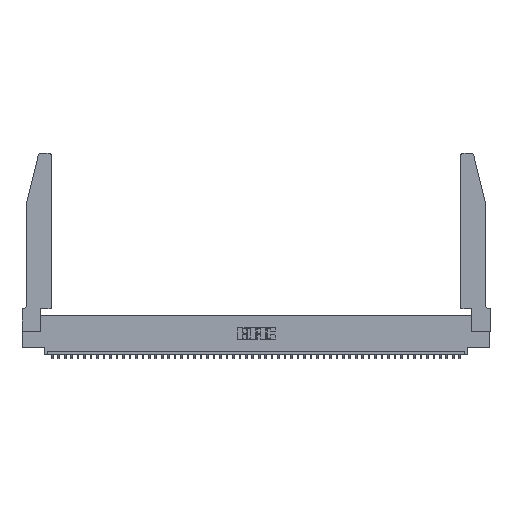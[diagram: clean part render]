
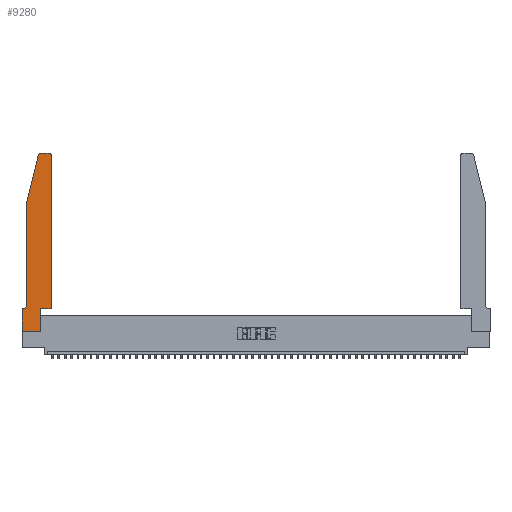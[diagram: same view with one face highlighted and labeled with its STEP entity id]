
A CAD part, top view. The second image highlights one B-rep face of the part: STEP entity #9280.
In plain terms, the highlighted planar face has unit normal (0, 0, 1).
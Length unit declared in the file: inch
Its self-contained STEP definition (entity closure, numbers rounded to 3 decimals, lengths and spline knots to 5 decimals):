
#1096 = ORIENTED_EDGE ( 'NONE', *, *, #9800, .T. ) ;
#2021 = EDGE_CURVE ( 'NONE', #10734, #32053, #25506, .T. ) ;
#2252 = EDGE_CURVE ( 'NONE', #7251, #27477, #3720, .T. ) ;
#2760 = VECTOR ( 'NONE', #45654, 39.37008 ) ;
#3720 = LINE ( 'NONE', #4627, #30350 ) ;
#4627 = CARTESIAN_POINT ( 'NONE',  ( 0.0755, 2., 0.37 ) ) ;
#4835 = ORIENTED_EDGE ( 'NONE', *, *, #45295, .T. ) ;
#5067 = ORIENTED_EDGE ( 'NONE', *, *, #29878, .T. ) ;
#5725 = EDGE_CURVE ( 'NONE', #32053, #15196, #8886, .T. ) ;
#6738 = ORIENTED_EDGE ( 'NONE', *, *, #2021, .T. ) ;
#7180 = DIRECTION ( 'NONE',  ( 1., 0., 0. ) ) ;
#7251 = VERTEX_POINT ( 'NONE', #35758 ) ;
#7427 = ORIENTED_EDGE ( 'NONE', *, *, #42457, .T. ) ;
#7876 = FACE_OUTER_BOUND ( 'NONE', #43813, .T. ) ;
#8027 = VERTEX_POINT ( 'NONE', #46887 ) ;
#8886 = LINE ( 'NONE', #47976, #35520 ) ;
#9280 = ADVANCED_FACE ( 'NONE', ( #7876 ), #30654, .T. ) ;
#9800 = EDGE_CURVE ( 'NONE', #8027, #15272, #48473, .T. ) ;
#9915 = CARTESIAN_POINT ( 'NONE',  ( 0.0055, 0.42, 0.37 ) ) ;
#10416 = CARTESIAN_POINT ( 'NONE',  ( 0.0755, 0.42, 0.37 ) ) ;
#10734 = VERTEX_POINT ( 'NONE', #34303 ) ;
#13925 = ORIENTED_EDGE ( 'NONE', *, *, #35368, .T. ) ;
#13956 = AXIS2_PLACEMENT_3D ( 'NONE', #34235, #45942, #7180 ) ;
#14145 = DIRECTION ( 'NONE',  ( 0., 0., -1. ) ) ;
#14603 = CARTESIAN_POINT ( 'NONE',  ( 0.4505, 2.72, 0.37 ) ) ;
#14678 = CARTESIAN_POINT ( 'NONE',  ( 0.2865, 0.35, 0.37 ) ) ;
#15196 = VERTEX_POINT ( 'NONE', #14603 ) ;
#15272 = VERTEX_POINT ( 'NONE', #49476 ) ;
#15698 = VERTEX_POINT ( 'NONE', #37585 ) ;
#16337 = AXIS2_PLACEMENT_3D ( 'NONE', #9915, #14145, #44931 ) ;
#16868 = DIRECTION ( 'NONE',  ( -1., 0., 0. ) ) ;
#17302 = VECTOR ( 'NONE', #46045, 39.37008 ) ;
#17576 = VECTOR ( 'NONE', #29086, 39.37008 ) ;
#19147 = LINE ( 'NONE', #33897, #37896 ) ;
#20569 = ORIENTED_EDGE ( 'NONE', *, *, #5725, .T. ) ;
#22042 = CARTESIAN_POINT ( 'NONE',  ( 0.4505, 0.35, 0.37 ) ) ;
#23129 = LINE ( 'NONE', #39863, #33415 ) ;
#23311 = CARTESIAN_POINT ( 'NONE',  ( 0.284, 2.72, 0.37 ) ) ;
#23325 = LINE ( 'NONE', #14678, #2760 ) ;
#23459 = EDGE_CURVE ( 'NONE', #35529, #7251, #48025, .T. ) ;
#24112 = ORIENTED_EDGE ( 'NONE', *, *, #24446, .T. ) ;
#24446 = EDGE_CURVE ( 'NONE', #15698, #35529, #23129, .T. ) ;
#24865 = CARTESIAN_POINT ( 'NONE',  ( 0.0755, 0.35, 0.37 ) ) ;
#25506 = LINE ( 'NONE', #34891, #44885 ) ;
#26017 = VECTOR ( 'NONE', #27885, 39.37008 ) ;
#26699 = CARTESIAN_POINT ( 'NONE',  ( 0.0755, 2., 0.37 ) ) ;
#26878 = CARTESIAN_POINT ( 'NONE',  ( 0., 0., 0.37 ) ) ;
#27252 = LINE ( 'NONE', #24865, #17576 ) ;
#27477 = VERTEX_POINT ( 'NONE', #35818 ) ;
#27521 = DIRECTION ( 'NONE',  ( 0., 0., 1. ) ) ;
#27621 = VERTEX_POINT ( 'NONE', #31876 ) ;
#27885 = DIRECTION ( 'NONE',  ( 0., -1., 0. ) ) ;
#28814 = DIRECTION ( 'NONE',  ( 0., 1., 0. ) ) ;
#29086 = DIRECTION ( 'NONE',  ( -1., 0., 0. ) ) ;
#29878 = EDGE_CURVE ( 'NONE', #27621, #8027, #27252, .T. ) ;
#29888 = ORIENTED_EDGE ( 'NONE', *, *, #41533, .T. ) ;
#30350 = VECTOR ( 'NONE', #36550, 39.37008 ) ;
#30654 = PLANE ( 'NONE',  #13956 ) ;
#31765 = AXIS2_PLACEMENT_3D ( 'NONE', #23311, #27521, #46859 ) ;
#31876 = CARTESIAN_POINT ( 'NONE',  ( 0.0055, 0.35, 0.37 ) ) ;
#32053 = VERTEX_POINT ( 'NONE', #22042 ) ;
#32510 = AXIS2_PLACEMENT_3D ( 'NONE', #35564, #43703, #43038 ) ;
#33281 = CIRCLE ( 'NONE', #16337, 0.07 ) ;
#33415 = VECTOR ( 'NONE', #16868, 39.37008 ) ;
#33557 = CARTESIAN_POINT ( 'NONE',  ( 0.284, 2.75, 0.37 ) ) ;
#33897 = CARTESIAN_POINT ( 'NONE',  ( 0., 0., 0.37 ) ) ;
#34235 = CARTESIAN_POINT ( 'NONE',  ( 0., 0.35, 0.37 ) ) ;
#34303 = CARTESIAN_POINT ( 'NONE',  ( 0.2865, 0.35, 0.37 ) ) ;
#34891 = CARTESIAN_POINT ( 'NONE',  ( 0.4505, 0.35, 0.37 ) ) ;
#35215 = DIRECTION ( 'NONE',  ( 1., 0., 0. ) ) ;
#35368 = EDGE_CURVE ( 'NONE', #35607, #27621, #33281, .T. ) ;
#35370 = VERTEX_POINT ( 'NONE', #36957 ) ;
#35520 = VECTOR ( 'NONE', #28814, 39.37008 ) ;
#35529 = VERTEX_POINT ( 'NONE', #33557 ) ;
#35564 = CARTESIAN_POINT ( 'NONE',  ( 0.4205, 2.72, 0.37 ) ) ;
#35607 = VERTEX_POINT ( 'NONE', #10416 ) ;
#35758 = CARTESIAN_POINT ( 'NONE',  ( 0.25487, 2.72718, 0.37 ) ) ;
#35818 = CARTESIAN_POINT ( 'NONE',  ( 0.0755, 2., 0.37 ) ) ;
#36550 = DIRECTION ( 'NONE',  ( -0.239, -0.971, 0. ) ) ;
#36957 = CARTESIAN_POINT ( 'NONE',  ( 0.2865, 0., 0.37 ) ) ;
#37585 = CARTESIAN_POINT ( 'NONE',  ( 0.4205, 2.75, 0.37 ) ) ;
#37746 = EDGE_CURVE ( 'NONE', #27477, #35607, #41480, .T. ) ;
#37896 = VECTOR ( 'NONE', #42175, 39.37008 ) ;
#39863 = CARTESIAN_POINT ( 'NONE',  ( 0.2605, 2.75, 0.37 ) ) ;
#41480 = LINE ( 'NONE', #26699, #17302 ) ;
#41533 = EDGE_CURVE ( 'NONE', #15272, #35370, #19147, .T. ) ;
#42175 = DIRECTION ( 'NONE',  ( 1., 0., 0. ) ) ;
#42290 = ORIENTED_EDGE ( 'NONE', *, *, #37746, .T. ) ;
#42457 = EDGE_CURVE ( 'NONE', #35370, #10734, #23325, .T. ) ;
#43038 = DIRECTION ( 'NONE',  ( 1., 0., 0. ) ) ;
#43703 = DIRECTION ( 'NONE',  ( 0., 0., 1. ) ) ;
#43813 = EDGE_LOOP ( 'NONE', ( #24112, #46047, #44762, #42290, #13925, #5067, #1096, #29888, #7427, #6738, #20569, #4835 ) ) ;
#44762 = ORIENTED_EDGE ( 'NONE', *, *, #2252, .T. ) ;
#44885 = VECTOR ( 'NONE', #35215, 39.37008 ) ;
#44931 = DIRECTION ( 'NONE',  ( -1., 0., 0. ) ) ;
#45295 = EDGE_CURVE ( 'NONE', #15196, #15698, #46049, .T. ) ;
#45654 = DIRECTION ( 'NONE',  ( 0., 1., 0. ) ) ;
#45942 = DIRECTION ( 'NONE',  ( 0., 0., 1. ) ) ;
#46045 = DIRECTION ( 'NONE',  ( 0., -1., 0. ) ) ;
#46047 = ORIENTED_EDGE ( 'NONE', *, *, #23459, .T. ) ;
#46049 = CIRCLE ( 'NONE', #32510, 0.03 ) ;
#46859 = DIRECTION ( 'NONE',  ( 1., 0., 0. ) ) ;
#46887 = CARTESIAN_POINT ( 'NONE',  ( 0., 0.35, 0.37 ) ) ;
#47976 = CARTESIAN_POINT ( 'NONE',  ( 0.4505, 0.35, 0.37 ) ) ;
#48025 = CIRCLE ( 'NONE', #31765, 0.03 ) ;
#48473 = LINE ( 'NONE', #26878, #26017 ) ;
#49476 = CARTESIAN_POINT ( 'NONE',  ( 0., 0., 0.37 ) ) ;
